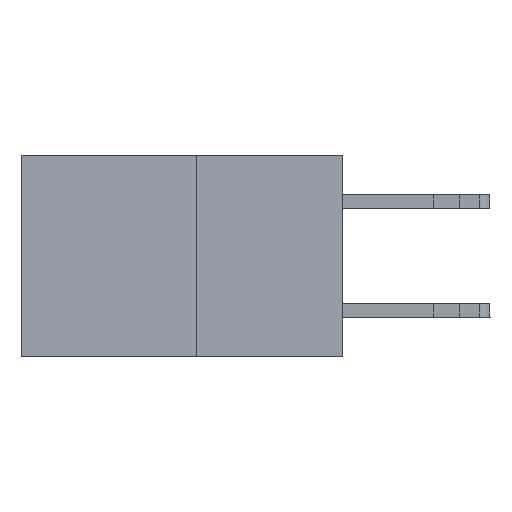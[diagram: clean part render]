
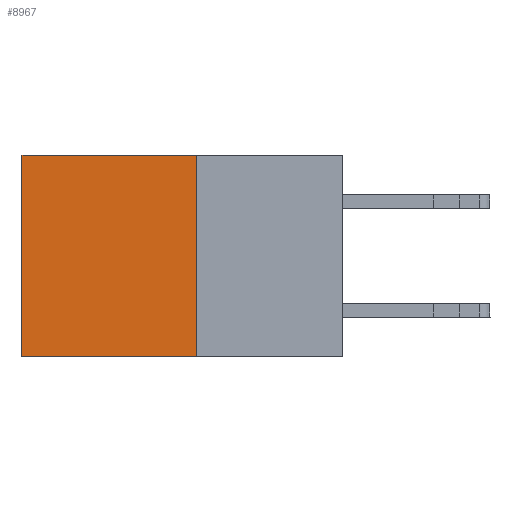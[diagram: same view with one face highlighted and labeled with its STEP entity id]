
A CAD part, left-side view. The second image highlights one B-rep face of the part: STEP entity #8967.
In plain terms, the highlighted planar face has unit normal (-1, 0, 0).
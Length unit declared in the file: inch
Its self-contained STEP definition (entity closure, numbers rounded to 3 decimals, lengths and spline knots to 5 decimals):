
#52 = LINE ( 'NONE', #30896, #25240 ) ;
#367 = DIRECTION ( 'NONE',  ( 1., 0., 0. ) ) ;
#1289 = CARTESIAN_POINT ( 'NONE',  ( 0.277, 0.59, -0.37 ) ) ;
#1348 = EDGE_CURVE ( 'NONE', #2238, #29747, #25238, .T. ) ;
#2238 = VERTEX_POINT ( 'NONE', #5847 ) ;
#3249 = VERTEX_POINT ( 'NONE', #3970 ) ;
#3628 = VECTOR ( 'NONE', #16247, 39.37008 ) ;
#3862 = DIRECTION ( 'NONE',  ( 0., 0., -1. ) ) ;
#3970 = CARTESIAN_POINT ( 'NONE',  ( 0.277, 0.59, -0.37 ) ) ;
#5356 = CARTESIAN_POINT ( 'NONE',  ( 0.277, 0.27, -0.37 ) ) ;
#5847 = CARTESIAN_POINT ( 'NONE',  ( 0.277, 0.27, 0. ) ) ;
#6115 = LINE ( 'NONE', #29349, #31977 ) ;
#8047 = ORIENTED_EDGE ( 'NONE', *, *, #14501, .F. ) ;
#8718 = CARTESIAN_POINT ( 'NONE',  ( 0.277, 0.27, -0.37 ) ) ;
#8967 = ADVANCED_FACE ( 'NONE', ( #12874 ), #30472, .F. ) ;
#11586 = EDGE_LOOP ( 'NONE', ( #16178, #8047, #20887, #16777 ) ) ;
#12874 = FACE_OUTER_BOUND ( 'NONE', #11586, .T. ) ;
#14474 = AXIS2_PLACEMENT_3D ( 'NONE', #5356, #367, #18001 ) ;
#14501 = EDGE_CURVE ( 'NONE', #29747, #3249, #6115, .T. ) ;
#14573 = LINE ( 'NONE', #1289, #26329 ) ;
#14578 = CARTESIAN_POINT ( 'NONE',  ( 0.277, 0.27, -0.37 ) ) ;
#16178 = ORIENTED_EDGE ( 'NONE', *, *, #26118, .T. ) ;
#16247 = DIRECTION ( 'NONE',  ( 0., 0., -1. ) ) ;
#16777 = ORIENTED_EDGE ( 'NONE', *, *, #17511, .T. ) ;
#16821 = DIRECTION ( 'NONE',  ( 0., 1., 0. ) ) ;
#17511 = EDGE_CURVE ( 'NONE', #2238, #28881, #52, .T. ) ;
#18001 = DIRECTION ( 'NONE',  ( 0., 0., -1. ) ) ;
#20887 = ORIENTED_EDGE ( 'NONE', *, *, #1348, .F. ) ;
#23452 = DIRECTION ( 'NONE',  ( 0., 1., 0. ) ) ;
#25238 = LINE ( 'NONE', #14578, #3628 ) ;
#25240 = VECTOR ( 'NONE', #23452, 39.37008 ) ;
#26118 = EDGE_CURVE ( 'NONE', #28881, #3249, #14573, .T. ) ;
#26329 = VECTOR ( 'NONE', #3862, 39.37008 ) ;
#28881 = VERTEX_POINT ( 'NONE', #30785 ) ;
#29349 = CARTESIAN_POINT ( 'NONE',  ( 0.277, 0.27, -0.37 ) ) ;
#29747 = VERTEX_POINT ( 'NONE', #8718 ) ;
#30472 = PLANE ( 'NONE',  #14474 ) ;
#30785 = CARTESIAN_POINT ( 'NONE',  ( 0.277, 0.59, 0. ) ) ;
#30896 = CARTESIAN_POINT ( 'NONE',  ( 0.277, 0.27, 0. ) ) ;
#31977 = VECTOR ( 'NONE', #16821, 39.37008 ) ;
